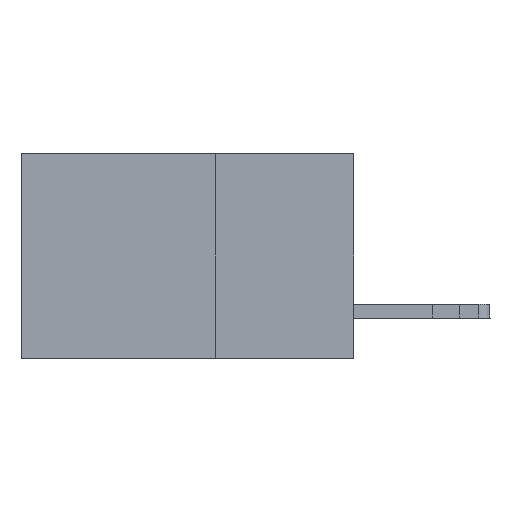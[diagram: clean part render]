
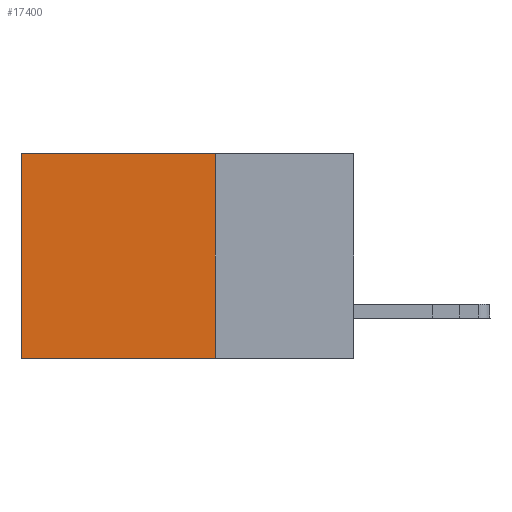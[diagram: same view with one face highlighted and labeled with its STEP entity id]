
A CAD part, left-side view. The second image highlights one B-rep face of the part: STEP entity #17400.
In plain terms, the highlighted planar face has unit normal (-1, 0, 0).
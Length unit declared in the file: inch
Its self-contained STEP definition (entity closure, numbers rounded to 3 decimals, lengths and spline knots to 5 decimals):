
#1627 = DIRECTION ( 'NONE',  ( 0., 1., 0. ) ) ;
#1690 = CARTESIAN_POINT ( 'NONE',  ( 0.2875, 0.6, 0. ) ) ;
#2281 = DIRECTION ( 'NONE',  ( 0., 0., -1. ) ) ;
#2872 = PLANE ( 'NONE',  #14190 ) ;
#3953 = VECTOR ( 'NONE', #1627, 39.37008 ) ;
#3981 = VECTOR ( 'NONE', #15789, 39.37008 ) ;
#4351 = EDGE_LOOP ( 'NONE', ( #16237, #8090, #22840, #6457 ) ) ;
#4614 = VERTEX_POINT ( 'NONE', #7151 ) ;
#4820 = DIRECTION ( 'NONE',  ( 0., 0., -1. ) ) ;
#5972 = EDGE_CURVE ( 'NONE', #19270, #9467, #19275, .T. ) ;
#6457 = ORIENTED_EDGE ( 'NONE', *, *, #8704, .T. ) ;
#7151 = CARTESIAN_POINT ( 'NONE',  ( 0.2875, 0.6, -0.37 ) ) ;
#7446 = CARTESIAN_POINT ( 'NONE',  ( 0.2875, 0.25, 0. ) ) ;
#8090 = ORIENTED_EDGE ( 'NONE', *, *, #20464, .F. ) ;
#8704 = EDGE_CURVE ( 'NONE', #19270, #24417, #14696, .T. ) ;
#9467 = VERTEX_POINT ( 'NONE', #11717 ) ;
#10506 = CARTESIAN_POINT ( 'NONE',  ( 0.2875, 0.25, 0. ) ) ;
#11717 = CARTESIAN_POINT ( 'NONE',  ( 0.2875, 0.25, -0.37 ) ) ;
#14190 = AXIS2_PLACEMENT_3D ( 'NONE', #10506, #16321, #4820 ) ;
#14696 = LINE ( 'NONE', #20747, #3953 ) ;
#15789 = DIRECTION ( 'NONE',  ( 0., 0., -1. ) ) ;
#16237 = ORIENTED_EDGE ( 'NONE', *, *, #17217, .T. ) ;
#16321 = DIRECTION ( 'NONE',  ( 1., 0., 0. ) ) ;
#16952 = VECTOR ( 'NONE', #2281, 39.37008 ) ;
#17217 = EDGE_CURVE ( 'NONE', #24417, #4614, #21953, .T. ) ;
#17400 = ADVANCED_FACE ( 'NONE', ( #23990 ), #2872, .F. ) ;
#18641 = CARTESIAN_POINT ( 'NONE',  ( 0.2875, 0.25, -0.37 ) ) ;
#18695 = VECTOR ( 'NONE', #24187, 39.37008 ) ;
#19270 = VERTEX_POINT ( 'NONE', #7446 ) ;
#19275 = LINE ( 'NONE', #24269, #3981 ) ;
#19490 = CARTESIAN_POINT ( 'NONE',  ( 0.2875, 0.6, 0. ) ) ;
#20464 = EDGE_CURVE ( 'NONE', #9467, #4614, #23646, .T. ) ;
#20747 = CARTESIAN_POINT ( 'NONE',  ( 0.2875, 0.25, 0. ) ) ;
#21953 = LINE ( 'NONE', #19490, #16952 ) ;
#22840 = ORIENTED_EDGE ( 'NONE', *, *, #5972, .F. ) ;
#23646 = LINE ( 'NONE', #18641, #18695 ) ;
#23990 = FACE_OUTER_BOUND ( 'NONE', #4351, .T. ) ;
#24187 = DIRECTION ( 'NONE',  ( 0., 1., 0. ) ) ;
#24269 = CARTESIAN_POINT ( 'NONE',  ( 0.2875, 0.25, 0. ) ) ;
#24417 = VERTEX_POINT ( 'NONE', #1690 ) ;
